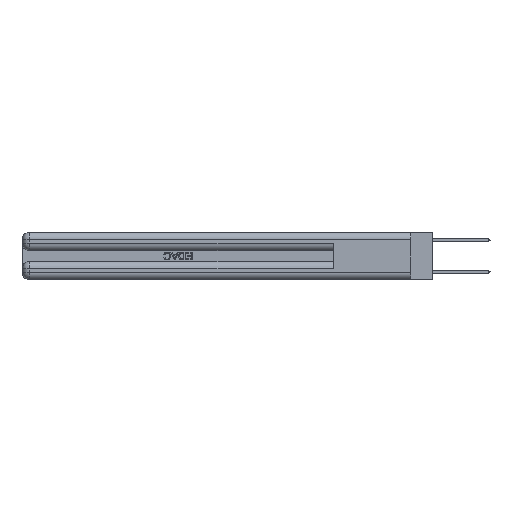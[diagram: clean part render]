
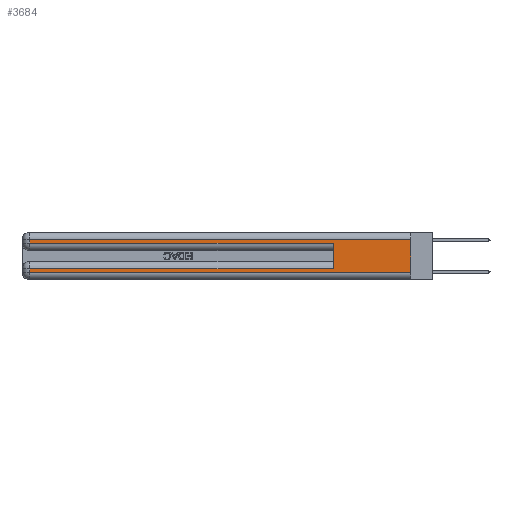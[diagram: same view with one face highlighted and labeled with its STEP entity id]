
A CAD part, left-side view. The second image highlights one B-rep face of the part: STEP entity #3684.
In plain terms, the highlighted planar face has unit normal (-1, 0, 0).
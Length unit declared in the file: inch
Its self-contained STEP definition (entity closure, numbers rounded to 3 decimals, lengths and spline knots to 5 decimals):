
#259 = CARTESIAN_POINT ( 'NONE',  ( 0., 2.94, 0.31 ) ) ;
#891 = CARTESIAN_POINT ( 'NONE',  ( 0., 0.6, 0.145 ) ) ;
#1482 = CARTESIAN_POINT ( 'NONE',  ( 0., 0., 0.31 ) ) ;
#1554 = VECTOR ( 'NONE', #33092, 39.37008 ) ;
#1690 = LINE ( 'NONE', #15213, #19458 ) ;
#2619 = VERTEX_POINT ( 'NONE', #19258 ) ;
#3007 = CARTESIAN_POINT ( 'NONE',  ( 0., 2.94, 0.37 ) ) ;
#3336 = EDGE_CURVE ( 'NONE', #26879, #2619, #22543, .T. ) ;
#3483 = CARTESIAN_POINT ( 'NONE',  ( 0., 0., 0.06 ) ) ;
#3514 = CARTESIAN_POINT ( 'NONE',  ( 0., 2.94, 0.06 ) ) ;
#3684 = ADVANCED_FACE ( 'NONE', ( #19183 ), #6166, .F. ) ;
#3703 = DIRECTION ( 'NONE',  ( 1., 0., 0. ) ) ;
#4225 = LINE ( 'NONE', #891, #5486 ) ;
#4354 = CARTESIAN_POINT ( 'NONE',  ( 0., 0., 0.285 ) ) ;
#5486 = VECTOR ( 'NONE', #22331, 39.37008 ) ;
#5966 = VECTOR ( 'NONE', #9156, 39.37008 ) ;
#6166 = PLANE ( 'NONE',  #24647 ) ;
#6242 = EDGE_LOOP ( 'NONE', ( #13770, #12661, #25315, #25892, #14727, #31530, #13344, #33815 ) ) ;
#7913 = LINE ( 'NONE', #3007, #18277 ) ;
#9141 = CARTESIAN_POINT ( 'NONE',  ( 0., 2.94, 0.37 ) ) ;
#9156 = DIRECTION ( 'NONE',  ( 0., 1., 0. ) ) ;
#9318 = CARTESIAN_POINT ( 'NONE',  ( 0., 0., 0.37 ) ) ;
#10758 = CARTESIAN_POINT ( 'NONE',  ( 0., 0.6, 0.285 ) ) ;
#11438 = LINE ( 'NONE', #9318, #1554 ) ;
#11894 = VECTOR ( 'NONE', #17883, 39.37008 ) ;
#12350 = DIRECTION ( 'NONE',  ( 0., 1., 0. ) ) ;
#12661 = ORIENTED_EDGE ( 'NONE', *, *, #21365, .T. ) ;
#13344 = ORIENTED_EDGE ( 'NONE', *, *, #31421, .T. ) ;
#13770 = ORIENTED_EDGE ( 'NONE', *, *, #22787, .F. ) ;
#14201 = EDGE_CURVE ( 'NONE', #30508, #22649, #20512, .T. ) ;
#14727 = ORIENTED_EDGE ( 'NONE', *, *, #24185, .F. ) ;
#14958 = VECTOR ( 'NONE', #19176, 39.37008 ) ;
#15213 = CARTESIAN_POINT ( 'NONE',  ( 0., 0., 0.06 ) ) ;
#15329 = CARTESIAN_POINT ( 'NONE',  ( 0., 0., 0.085 ) ) ;
#16900 = CARTESIAN_POINT ( 'NONE',  ( 0., 0., 0.37 ) ) ;
#17347 = CARTESIAN_POINT ( 'NONE',  ( 0., 2.94, 0.285 ) ) ;
#17883 = DIRECTION ( 'NONE',  ( 0., -1., 0. ) ) ;
#18277 = VECTOR ( 'NONE', #18820, 39.37008 ) ;
#18820 = DIRECTION ( 'NONE',  ( 0., 0., -1. ) ) ;
#19176 = DIRECTION ( 'NONE',  ( 0., 0., -1. ) ) ;
#19183 = FACE_OUTER_BOUND ( 'NONE', #6242, .T. ) ;
#19258 = CARTESIAN_POINT ( 'NONE',  ( 0., 2.94, 0.085 ) ) ;
#19458 = VECTOR ( 'NONE', #31068, 39.37008 ) ;
#19881 = VERTEX_POINT ( 'NONE', #3483 ) ;
#20512 = LINE ( 'NONE', #4354, #11894 ) ;
#21365 = EDGE_CURVE ( 'NONE', #26736, #25290, #25858, .T. ) ;
#21853 = EDGE_CURVE ( 'NONE', #28974, #19881, #1690, .T. ) ;
#22331 = DIRECTION ( 'NONE',  ( 0., 0., 1. ) ) ;
#22510 = CARTESIAN_POINT ( 'NONE',  ( 0., 0., 0.31 ) ) ;
#22543 = LINE ( 'NONE', #15329, #22924 ) ;
#22649 = VERTEX_POINT ( 'NONE', #10758 ) ;
#22787 = EDGE_CURVE ( 'NONE', #26736, #19881, #11438, .T. ) ;
#22924 = VECTOR ( 'NONE', #12350, 39.37008 ) ;
#24185 = EDGE_CURVE ( 'NONE', #26879, #22649, #4225, .T. ) ;
#24647 = AXIS2_PLACEMENT_3D ( 'NONE', #16900, #3703, #29940 ) ;
#25290 = VERTEX_POINT ( 'NONE', #259 ) ;
#25315 = ORIENTED_EDGE ( 'NONE', *, *, #28783, .T. ) ;
#25858 = LINE ( 'NONE', #22510, #5966 ) ;
#25892 = ORIENTED_EDGE ( 'NONE', *, *, #14201, .T. ) ;
#26736 = VERTEX_POINT ( 'NONE', #1482 ) ;
#26879 = VERTEX_POINT ( 'NONE', #34020 ) ;
#28783 = EDGE_CURVE ( 'NONE', #25290, #30508, #7913, .T. ) ;
#28974 = VERTEX_POINT ( 'NONE', #3514 ) ;
#29940 = DIRECTION ( 'NONE',  ( 0., 0., -1. ) ) ;
#30508 = VERTEX_POINT ( 'NONE', #17347 ) ;
#31068 = DIRECTION ( 'NONE',  ( 0., -1., 0. ) ) ;
#31421 = EDGE_CURVE ( 'NONE', #2619, #28974, #33264, .T. ) ;
#31530 = ORIENTED_EDGE ( 'NONE', *, *, #3336, .T. ) ;
#33092 = DIRECTION ( 'NONE',  ( 0., 0., -1. ) ) ;
#33264 = LINE ( 'NONE', #9141, #14958 ) ;
#33815 = ORIENTED_EDGE ( 'NONE', *, *, #21853, .T. ) ;
#34020 = CARTESIAN_POINT ( 'NONE',  ( 0., 0.6, 0.085 ) ) ;
